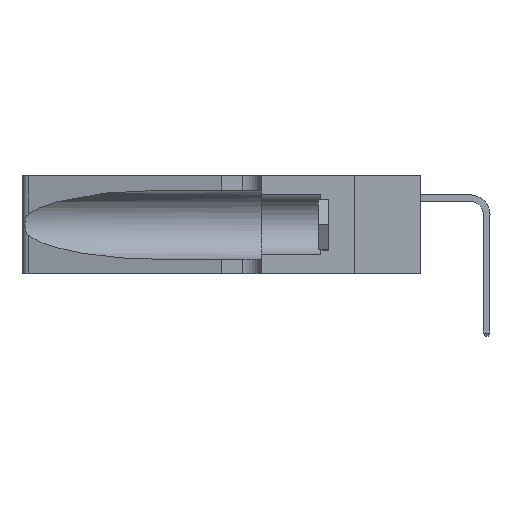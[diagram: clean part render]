
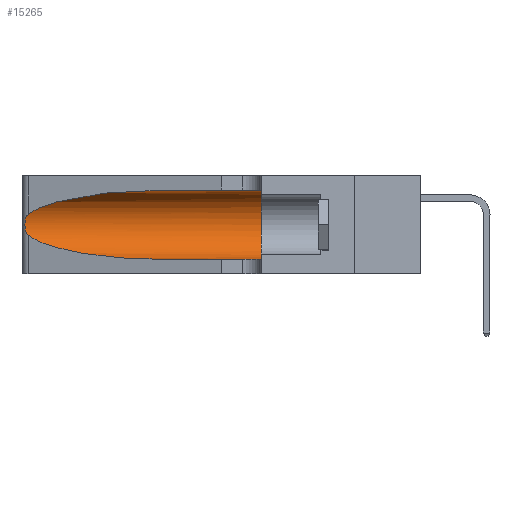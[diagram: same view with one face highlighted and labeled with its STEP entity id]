
A CAD part, left-side view. The second image highlights one B-rep face of the part: STEP entity #15265.
In plain terms, the highlighted cylindrical face has radius 3.308 mm (diameter 6.617 mm), a partial arc.
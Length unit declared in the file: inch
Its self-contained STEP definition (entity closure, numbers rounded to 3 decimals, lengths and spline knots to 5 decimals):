
#116 = ORIENTED_EDGE ( 'NONE', *, *, #12308, .T. ) ;
#317 = DIRECTION ( 'NONE',  ( 0., -1., 0. ) ) ;
#542 = CARTESIAN_POINT ( 'NONE',  ( 0.25555, 1.22994, 0.2215 ) ) ;
#626 = CARTESIAN_POINT ( 'NONE',  ( 0.26018, 1.23835, 0.19895 ) ) ;
#648 = ORIENTED_EDGE ( 'NONE', *, *, #19867, .F. ) ;
#1263 = CARTESIAN_POINT ( 'NONE',  ( 0.25487, 1.22718, 0.14631 ) ) ;
#1796 = CARTESIAN_POINT ( 'NONE',  ( 0.1305, 0.35, 0.05475 ) ) ;
#1943 =( BOUNDED_CURVE ( )  B_SPLINE_CURVE ( 3, ( #12297, #4451, #18215, #6495 ),
 .UNSPECIFIED., .F., .T. ) 
 B_SPLINE_CURVE_WITH_KNOTS ( ( 4, 4 ),
 ( 1.5708, 2.84003 ),
 .UNSPECIFIED. ) 
 CURVE ( )  GEOMETRIC_REPRESENTATION_ITEM ( )  RATIONAL_B_SPLINE_CURVE ( ( 1., 0.87, 0.87, 1. ) ) 
 REPRESENTATION_ITEM ( '' )  );
#2592 = CARTESIAN_POINT ( 'NONE',  ( 0.26075, 1.23896, 0.178 ) ) ;
#3121 = ORIENTED_EDGE ( 'NONE', *, *, #17012, .T. ) ;
#4451 = CARTESIAN_POINT ( 'NONE',  ( 0.18966, 0.96281, 0.31525 ) ) ;
#4512 = VERTEX_POINT ( 'NONE', #12174 ) ;
#4556 = CARTESIAN_POINT ( 'NONE',  ( 0.25856, 1.23593, 0.16098 ) ) ;
#4584 = CARTESIAN_POINT ( 'NONE',  ( 0.1305, 0.72297, 0.05475 ) ) ;
#5103 = VERTEX_POINT ( 'NONE', #19834 ) ;
#5215 = CYLINDRICAL_SURFACE ( 'NONE', #19100, 0.13025 ) ;
#5975 = EDGE_CURVE ( 'NONE', #22806, #4512, #1943, .T. ) ;
#6190 = VECTOR ( 'NONE', #317, 39.37008 ) ;
#6208 = EDGE_CURVE ( 'NONE', #10351, #16423, #22727, .T. ) ;
#6495 = CARTESIAN_POINT ( 'NONE',  ( 0.25487, 1.22718, 0.22369 ) ) ;
#6517 = CARTESIAN_POINT ( 'NONE',  ( 0.25639, 1.23186, 0.15144 ) ) ;
#6811 = LINE ( 'NONE', #9962, #6190 ) ;
#7199 = DIRECTION ( 'NONE',  ( 0., 1., 0. ) ) ;
#7355 = EDGE_LOOP ( 'NONE', ( #18946, #3121, #10873, #116, #16922, #648 ) ) ;
#7513 = VECTOR ( 'NONE', #8671, 39.37008 ) ;
#7616 = CARTESIAN_POINT ( 'NONE',  ( 0.25487, 1.22718, 0.14631 ) ) ;
#8485 = CARTESIAN_POINT ( 'NONE',  ( 0.25487, 1.22718, 0.14631 ) ) ;
#8671 = DIRECTION ( 'NONE',  ( 0., -1., 0. ) ) ;
#9962 = CARTESIAN_POINT ( 'NONE',  ( 0.1305, 1.61858, 0.31525 ) ) ;
#10351 = VERTEX_POINT ( 'NONE', #7616 ) ;
#10355 = CARTESIAN_POINT ( 'NONE',  ( 0.25639, 1.23184, 0.21858 ) ) ;
#10425 = CARTESIAN_POINT ( 'NONE',  ( 0.1305, 0.72297, 0.31525 ) ) ;
#10682 = CARTESIAN_POINT ( 'NONE',  ( 0.1305, 1.61858, 0.185 ) ) ;
#10873 = ORIENTED_EDGE ( 'NONE', *, *, #6208, .T. ) ;
#10989 = CARTESIAN_POINT ( 'NONE',  ( 0.18966, 0.96281, 0.05475 ) ) ;
#12174 = CARTESIAN_POINT ( 'NONE',  ( 0.25487, 1.22718, 0.22369 ) ) ;
#12297 = CARTESIAN_POINT ( 'NONE',  ( 0.1305, 0.72297, 0.31525 ) ) ;
#12308 = EDGE_CURVE ( 'NONE', #16423, #20744, #23038, .T. ) ;
#12321 = CARTESIAN_POINT ( 'NONE',  ( 0.25854, 1.2359, 0.20912 ) ) ;
#12963 = CARTESIAN_POINT ( 'NONE',  ( 0.2373, 1.15595, 0.08982 ) ) ;
#14276 = CARTESIAN_POINT ( 'NONE',  ( 0.26075, 1.23896, 0.19203 ) ) ;
#14906 = CARTESIAN_POINT ( 'NONE',  ( 0.1305, 0.72297, 0.05475 ) ) ;
#15265 = ADVANCED_FACE ( 'NONE', ( #20768 ), #5215, .F. ) ;
#16236 = CARTESIAN_POINT ( 'NONE',  ( 0.26017, 1.23833, 0.17102 ) ) ;
#16423 = VERTEX_POINT ( 'NONE', #4584 ) ;
#16922 = ORIENTED_EDGE ( 'NONE', *, *, #20228, .F. ) ;
#17012 = EDGE_CURVE ( 'NONE', #4512, #10351, #20550, .T. ) ;
#18143 = CARTESIAN_POINT ( 'NONE',  ( 0.25487, 1.22718, 0.22369 ) ) ;
#18215 = CARTESIAN_POINT ( 'NONE',  ( 0.2373, 1.15595, 0.28018 ) ) ;
#18232 = CARTESIAN_POINT ( 'NONE',  ( 0.25789, 1.23486, 0.15765 ) ) ;
#18405 = CARTESIAN_POINT ( 'NONE',  ( 0.1305, 1.61858, 0.05475 ) ) ;
#18411 = CIRCLE ( 'NONE', #22594, 0.13025 ) ;
#18905 = CARTESIAN_POINT ( 'NONE',  ( 0.1305, 0.35, 0.185 ) ) ;
#18946 = ORIENTED_EDGE ( 'NONE', *, *, #5975, .T. ) ;
#19100 = AXIS2_PLACEMENT_3D ( 'NONE', #10682, #24259, #22344 ) ;
#19834 = CARTESIAN_POINT ( 'NONE',  ( 0.1305, 0.35, 0.31525 ) ) ;
#19867 = EDGE_CURVE ( 'NONE', #22806, #5103, #6811, .T. ) ;
#20167 = CARTESIAN_POINT ( 'NONE',  ( 0.25555, 1.22993, 0.14849 ) ) ;
#20228 = EDGE_CURVE ( 'NONE', #5103, #20744, #18411, .T. ) ;
#20550 = B_SPLINE_CURVE_WITH_KNOTS ( 'NONE', 3,
 ( #18143, #542, #10355, #23944, #12321, #626, #14276, #2592, #16236, #4556, #18232, #6517, #20167, #8485 ),
 .UNSPECIFIED., .F., .F.,
 ( 4, 2, 2, 2, 2, 2, 4 ),
 ( 0., 0.00027, 0.00053, 0.00107, 0.0016, 0.00187, 0.00214 ),
 .UNSPECIFIED. ) ;
#20744 = VERTEX_POINT ( 'NONE', #1796 ) ;
#20768 = FACE_OUTER_BOUND ( 'NONE', #7355, .T. ) ;
#20825 = DIRECTION ( 'NONE',  ( 0., 0., 1. ) ) ;
#22344 = DIRECTION ( 'NONE',  ( 0., 0., -1. ) ) ;
#22594 = AXIS2_PLACEMENT_3D ( 'NONE', #18905, #7199, #20825 ) ;
#22727 =( BOUNDED_CURVE ( )  B_SPLINE_CURVE ( 3, ( #1263, #12963, #10989, #14906 ),
 .UNSPECIFIED., .F., .T. ) 
 B_SPLINE_CURVE_WITH_KNOTS ( ( 4, 4 ),
 ( 3.44316, 4.71239 ),
 .UNSPECIFIED. ) 
 CURVE ( )  GEOMETRIC_REPRESENTATION_ITEM ( )  RATIONAL_B_SPLINE_CURVE ( ( 1., 0.87, 0.87, 1. ) ) 
 REPRESENTATION_ITEM ( '' )  );
#22806 = VERTEX_POINT ( 'NONE', #10425 ) ;
#23038 = LINE ( 'NONE', #18405, #7513 ) ;
#23944 = CARTESIAN_POINT ( 'NONE',  ( 0.25787, 1.23484, 0.2124 ) ) ;
#24259 = DIRECTION ( 'NONE',  ( 0., -1., 0. ) ) ;
